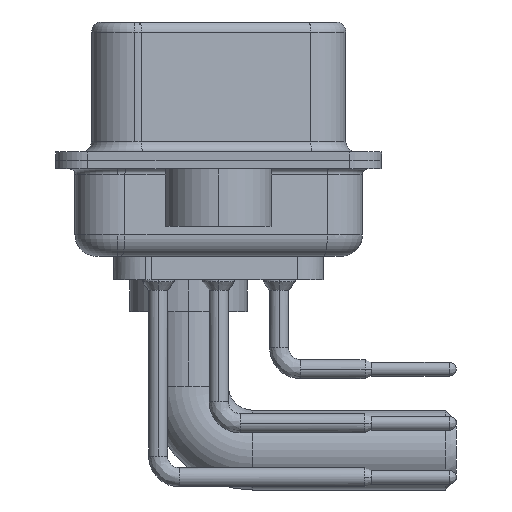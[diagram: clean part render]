
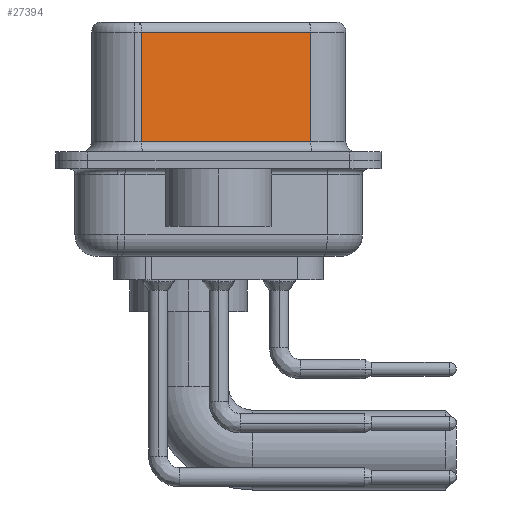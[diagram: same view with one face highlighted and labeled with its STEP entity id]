
A CAD part, left-side view. The second image highlights one B-rep face of the part: STEP entity #27394.
In plain terms, the highlighted planar face has unit normal (-0.985, -0.174, 0).
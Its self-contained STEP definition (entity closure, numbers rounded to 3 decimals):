
#195 = CARTESIAN_POINT ( 'NONE',  ( 3.73, 3.628, 6.02 ) ) ;
#436 = CARTESIAN_POINT ( 'NONE',  ( 5.132, -4.322, 6.02 ) ) ;
#664 = VECTOR ( 'NONE', #21745, 1000. ) ;
#5578 = DIRECTION ( 'NONE',  ( 0.985, 0.174, 0. ) ) ;
#5756 = FACE_OUTER_BOUND ( 'NONE', #10381, .T. ) ;
#5938 = LINE ( 'NONE', #436, #14447 ) ;
#6068 = CARTESIAN_POINT ( 'NONE',  ( 5.132, -4.322, 6.02 ) ) ;
#7963 = CARTESIAN_POINT ( 'NONE',  ( 5.132, -4.322, 6.52 ) ) ;
#8628 = DIRECTION ( 'NONE',  ( 0., 0., -1. ) ) ;
#9148 = EDGE_CURVE ( 'NONE', #16463, #12693, #19304, .T. ) ;
#10381 = EDGE_LOOP ( 'NONE', ( #27708, #30537, #31493, #29305 ) ) ;
#12693 = VERTEX_POINT ( 'NONE', #13344 ) ;
#13121 = EDGE_CURVE ( 'NONE', #24963, #35749, #13655, .T. ) ;
#13344 = CARTESIAN_POINT ( 'NONE',  ( 3.73, 3.628, 0.9 ) ) ;
#13655 = LINE ( 'NONE', #7963, #21597 ) ;
#14447 = VECTOR ( 'NONE', #20096, 1000. ) ;
#16463 = VERTEX_POINT ( 'NONE', #195 ) ;
#16539 = EDGE_CURVE ( 'NONE', #12693, #35749, #28460, .T. ) ;
#16961 = DIRECTION ( 'NONE',  ( -0.174, 0.985, 0. ) ) ;
#19304 = LINE ( 'NONE', #33947, #23757 ) ;
#20096 = DIRECTION ( 'NONE',  ( -0.174, 0.985, 0. ) ) ;
#20838 = AXIS2_PLACEMENT_3D ( 'NONE', #22476, #5578, #16961 ) ;
#21597 = VECTOR ( 'NONE', #24678, 1000. ) ;
#21745 = DIRECTION ( 'NONE',  ( 0.174, -0.985, 0. ) ) ;
#22423 = CARTESIAN_POINT ( 'NONE',  ( 5.132, -4.322, 0.9 ) ) ;
#22476 = CARTESIAN_POINT ( 'NONE',  ( 5.132, -4.322, 6.52 ) ) ;
#23757 = VECTOR ( 'NONE', #8628, 1000. ) ;
#24678 = DIRECTION ( 'NONE',  ( 0., 0., -1. ) ) ;
#24963 = VERTEX_POINT ( 'NONE', #6068 ) ;
#27394 = ADVANCED_FACE ( 'NONE', ( #5756 ), #30725, .F. ) ;
#27708 = ORIENTED_EDGE ( 'NONE', *, *, #13121, .F. ) ;
#28460 = LINE ( 'NONE', #22423, #664 ) ;
#28841 = CARTESIAN_POINT ( 'NONE',  ( 5.132, -4.322, 0.9 ) ) ;
#28876 = EDGE_CURVE ( 'NONE', #24963, #16463, #5938, .T. ) ;
#29305 = ORIENTED_EDGE ( 'NONE', *, *, #16539, .T. ) ;
#30537 = ORIENTED_EDGE ( 'NONE', *, *, #28876, .T. ) ;
#30725 = PLANE ( 'NONE',  #20838 ) ;
#31493 = ORIENTED_EDGE ( 'NONE', *, *, #9148, .T. ) ;
#33947 = CARTESIAN_POINT ( 'NONE',  ( 3.73, 3.628, 6.52 ) ) ;
#35749 = VERTEX_POINT ( 'NONE', #28841 ) ;
